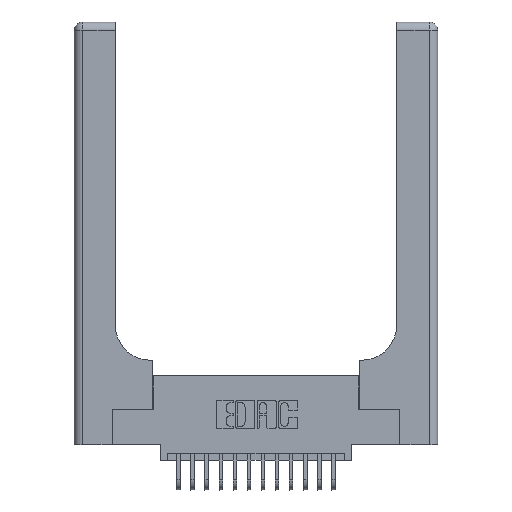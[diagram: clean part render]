
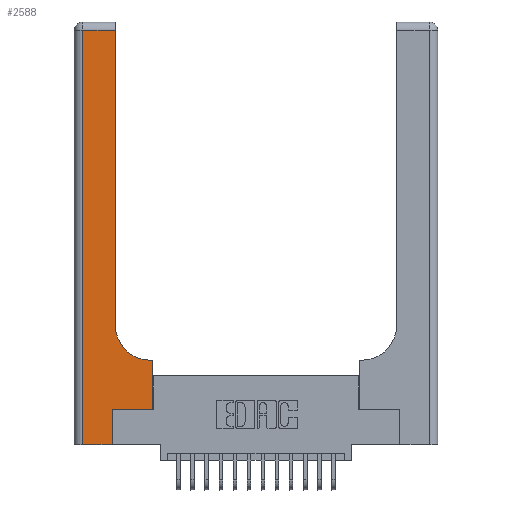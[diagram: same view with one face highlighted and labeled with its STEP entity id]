
A CAD part, top view. The second image highlights one B-rep face of the part: STEP entity #2588.
In plain terms, the highlighted planar face has unit normal (0, 0, 1).
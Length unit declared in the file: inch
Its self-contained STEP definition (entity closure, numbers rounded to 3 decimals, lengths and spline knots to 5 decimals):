
#243 = DIRECTION ( 'NONE',  ( -1., 0., 0. ) ) ;
#298 = VECTOR ( 'NONE', #17190, 39.37008 ) ;
#360 = DIRECTION ( 'NONE',  ( 1., 0., 0. ) ) ;
#519 = EDGE_CURVE ( 'NONE', #4628, #4224, #4341, .T. ) ;
#746 = VECTOR ( 'NONE', #17740, 39.37008 ) ;
#950 = EDGE_CURVE ( 'NONE', #5968, #9803, #17928, .T. ) ;
#1236 = VERTEX_POINT ( 'NONE', #11396 ) ;
#1274 = CARTESIAN_POINT ( 'NONE',  ( 0.5415, 0.6, 0.37 ) ) ;
#1718 = EDGE_LOOP ( 'NONE', ( #6745, #13568, #3805, #6926, #11477, #3929, #20048, #10128, #12809 ) ) ;
#1735 = EDGE_CURVE ( 'NONE', #5145, #5746, #11971, .T. ) ;
#2289 = EDGE_CURVE ( 'NONE', #4224, #5145, #5297, .T. ) ;
#2355 = VECTOR ( 'NONE', #243, 39.37008 ) ;
#2588 = ADVANCED_FACE ( 'NONE', ( #8979 ), #6217, .F. ) ;
#2760 = CARTESIAN_POINT ( 'NONE',  ( 0.269, 0.25, 0.37 ) ) ;
#3089 = CARTESIAN_POINT ( 'NONE',  ( 0.06, 3., 0.37 ) ) ;
#3740 = CARTESIAN_POINT ( 'NONE',  ( 0.2915, 3., 0.37 ) ) ;
#3805 = ORIENTED_EDGE ( 'NONE', *, *, #17315, .T. ) ;
#3929 = ORIENTED_EDGE ( 'NONE', *, *, #12325, .T. ) ;
#4224 = VERTEX_POINT ( 'NONE', #9690 ) ;
#4270 = LINE ( 'NONE', #15615, #298 ) ;
#4341 = LINE ( 'NONE', #15763, #9031 ) ;
#4562 = LINE ( 'NONE', #5295, #16163 ) ;
#4628 = VERTEX_POINT ( 'NONE', #14127 ) ;
#5099 = CARTESIAN_POINT ( 'NONE',  ( 0.269, 0.25, 0.37 ) ) ;
#5145 = VERTEX_POINT ( 'NONE', #1274 ) ;
#5295 = CARTESIAN_POINT ( 'NONE',  ( 0., 0., 0.37 ) ) ;
#5297 = LINE ( 'NONE', #16172, #2355 ) ;
#5430 = VERTEX_POINT ( 'NONE', #15187 ) ;
#5746 = VERTEX_POINT ( 'NONE', #7070 ) ;
#5968 = VERTEX_POINT ( 'NONE', #13649 ) ;
#6217 = PLANE ( 'NONE',  #18321 ) ;
#6528 = EDGE_CURVE ( 'NONE', #9969, #5430, #4270, .T. ) ;
#6702 = DIRECTION ( 'NONE',  ( 1., 0., 0. ) ) ;
#6745 = ORIENTED_EDGE ( 'NONE', *, *, #12206, .T. ) ;
#6926 = ORIENTED_EDGE ( 'NONE', *, *, #14710, .T. ) ;
#7070 = CARTESIAN_POINT ( 'NONE',  ( 0.2915, 0.85, 0.37 ) ) ;
#7820 = DIRECTION ( 'NONE',  ( -1., 0., 0. ) ) ;
#8979 = FACE_OUTER_BOUND ( 'NONE', #1718, .T. ) ;
#9031 = VECTOR ( 'NONE', #12639, 39.37008 ) ;
#9119 = DIRECTION ( 'NONE',  ( 0., 0., -1. ) ) ;
#9298 = CARTESIAN_POINT ( 'NONE',  ( 0.269, 0., 0.37 ) ) ;
#9690 = CARTESIAN_POINT ( 'NONE',  ( 0.5585, 0.6, 0.37 ) ) ;
#9803 = VERTEX_POINT ( 'NONE', #2760 ) ;
#9824 = DIRECTION ( 'NONE',  ( 0., 0., -1. ) ) ;
#9969 = VERTEX_POINT ( 'NONE', #11296 ) ;
#10120 = LINE ( 'NONE', #5099, #19743 ) ;
#10128 = ORIENTED_EDGE ( 'NONE', *, *, #2289, .T. ) ;
#10748 = VECTOR ( 'NONE', #20310, 39.37008 ) ;
#11296 = CARTESIAN_POINT ( 'NONE',  ( 0.2915, 2.94, 0.37 ) ) ;
#11396 = CARTESIAN_POINT ( 'NONE',  ( 0.06, 0., 0.37 ) ) ;
#11477 = ORIENTED_EDGE ( 'NONE', *, *, #950, .T. ) ;
#11613 = AXIS2_PLACEMENT_3D ( 'NONE', #19283, #9824, #360 ) ;
#11971 = CIRCLE ( 'NONE', #11613, 0.25 ) ;
#12206 = EDGE_CURVE ( 'NONE', #5746, #9969, #17519, .T. ) ;
#12235 = CARTESIAN_POINT ( 'NONE',  ( 0., 3., 0.37 ) ) ;
#12325 = EDGE_CURVE ( 'NONE', #9803, #4628, #10120, .T. ) ;
#12639 = DIRECTION ( 'NONE',  ( 0., 1., 0. ) ) ;
#12809 = ORIENTED_EDGE ( 'NONE', *, *, #1735, .T. ) ;
#13568 = ORIENTED_EDGE ( 'NONE', *, *, #6528, .T. ) ;
#13649 = CARTESIAN_POINT ( 'NONE',  ( 0.269, 0., 0.37 ) ) ;
#14079 = DIRECTION ( 'NONE',  ( 0., -1., 0. ) ) ;
#14127 = CARTESIAN_POINT ( 'NONE',  ( 0.5585, 0.25, 0.37 ) ) ;
#14710 = EDGE_CURVE ( 'NONE', #1236, #5968, #4562, .T. ) ;
#15187 = CARTESIAN_POINT ( 'NONE',  ( 0.06, 2.94, 0.37 ) ) ;
#15306 = VECTOR ( 'NONE', #14079, 39.37008 ) ;
#15615 = CARTESIAN_POINT ( 'NONE',  ( 0., 2.94, 0.37 ) ) ;
#15763 = CARTESIAN_POINT ( 'NONE',  ( 0.5585, 0.25, 0.37 ) ) ;
#16163 = VECTOR ( 'NONE', #16330, 39.37008 ) ;
#16172 = CARTESIAN_POINT ( 'NONE',  ( 0.2915, 0.6, 0.37 ) ) ;
#16330 = DIRECTION ( 'NONE',  ( 1., 0., 0. ) ) ;
#16839 = LINE ( 'NONE', #3089, #15306 ) ;
#17190 = DIRECTION ( 'NONE',  ( -1., 0., 0. ) ) ;
#17315 = EDGE_CURVE ( 'NONE', #5430, #1236, #16839, .T. ) ;
#17519 = LINE ( 'NONE', #3740, #746 ) ;
#17740 = DIRECTION ( 'NONE',  ( 0., 1., 0. ) ) ;
#17928 = LINE ( 'NONE', #9298, #10748 ) ;
#18321 = AXIS2_PLACEMENT_3D ( 'NONE', #12235, #9119, #7820 ) ;
#19283 = CARTESIAN_POINT ( 'NONE',  ( 0.5415, 0.85, 0.37 ) ) ;
#19743 = VECTOR ( 'NONE', #6702, 39.37008 ) ;
#20048 = ORIENTED_EDGE ( 'NONE', *, *, #519, .T. ) ;
#20310 = DIRECTION ( 'NONE',  ( 0., 1., 0. ) ) ;
